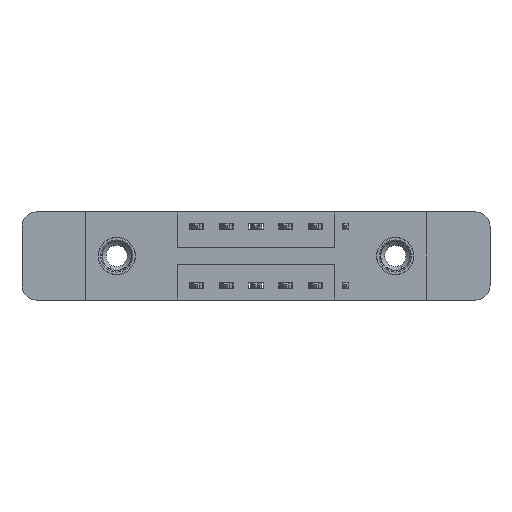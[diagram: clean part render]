
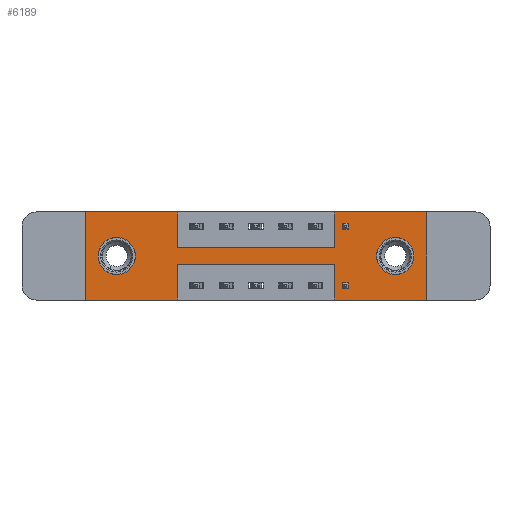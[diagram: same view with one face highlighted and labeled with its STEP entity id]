
A CAD part, front view. The second image highlights one B-rep face of the part: STEP entity #6189.
In plain terms, the highlighted planar face has unit normal (0, -1, 0).
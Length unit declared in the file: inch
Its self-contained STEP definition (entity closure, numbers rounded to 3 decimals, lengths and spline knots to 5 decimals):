
#10 = VERTEX_POINT ( 'NONE', #11869 ) ;
#125 = VECTOR ( 'NONE', #12789, 39.37008 ) ;
#380 = EDGE_CURVE ( 'NONE', #10252, #10491, #4422, .T. ) ;
#447 = EDGE_CURVE ( 'NONE', #5272, #11080, #8510, .T. ) ;
#458 = EDGE_CURVE ( 'NONE', #12099, #11880, #6457, .T. ) ;
#589 = EDGE_CURVE ( 'NONE', #10491, #10252, #1024, .T. ) ;
#596 = ORIENTED_EDGE ( 'NONE', *, *, #3957, .T. ) ;
#652 = CARTESIAN_POINT ( 'NONE',  ( 1.435, 0., -0.37 ) ) ;
#696 = EDGE_LOOP ( 'NONE', ( #4927, #13504, #6667, #5332, #2141, #5871, #3290, #5049, #10887, #3075, #12571, #9923 ) ) ;
#860 = CARTESIAN_POINT ( 'NONE',  ( 1.3025, 0., -0.185 ) ) ;
#926 = CIRCLE ( 'NONE', #1399, 0.078 ) ;
#971 = ORIENTED_EDGE ( 'NONE', *, *, #3456, .T. ) ;
#1024 = CIRCLE ( 'NONE', #1711, 0.078 ) ;
#1135 = CARTESIAN_POINT ( 'NONE',  ( 0.1325, 0., -0.263 ) ) ;
#1215 = VECTOR ( 'NONE', #3801, 39.37008 ) ;
#1244 = CARTESIAN_POINT ( 'NONE',  ( 1.0475, 0., -0.37 ) ) ;
#1246 = AXIS2_PLACEMENT_3D ( 'NONE', #860, #3007, #13574 ) ;
#1248 = CARTESIAN_POINT ( 'NONE',  ( 0., 0., 0. ) ) ;
#1298 = VECTOR ( 'NONE', #4616, 39.37008 ) ;
#1399 = AXIS2_PLACEMENT_3D ( 'NONE', #7793, #7524, #12070 ) ;
#1448 = EDGE_CURVE ( 'NONE', #11471, #2522, #7578, .T. ) ;
#1578 = VERTEX_POINT ( 'NONE', #8200 ) ;
#1674 = CARTESIAN_POINT ( 'NONE',  ( 1.0475, 0., 0. ) ) ;
#1711 = AXIS2_PLACEMENT_3D ( 'NONE', #5689, #4480, #12066 ) ;
#2111 = VECTOR ( 'NONE', #12059, 39.37008 ) ;
#2141 = ORIENTED_EDGE ( 'NONE', *, *, #9659, .F. ) ;
#2290 = DIRECTION ( 'NONE',  ( 0., 0., -1. ) ) ;
#2362 = LINE ( 'NONE', #5828, #8233 ) ;
#2522 = VERTEX_POINT ( 'NONE', #4399 ) ;
#2550 = EDGE_CURVE ( 'NONE', #9935, #12099, #9894, .T. ) ;
#2562 = EDGE_LOOP ( 'NONE', ( #596, #971 ) ) ;
#2643 = VECTOR ( 'NONE', #13912, 39.37008 ) ;
#2678 = VECTOR ( 'NONE', #2910, 39.37008 ) ;
#2857 = VECTOR ( 'NONE', #3156, 39.37008 ) ;
#2876 = EDGE_CURVE ( 'NONE', #11080, #3169, #6768, .T. ) ;
#2910 = DIRECTION ( 'NONE',  ( 0., 0., -1. ) ) ;
#3007 = DIRECTION ( 'NONE',  ( 0., 1., 0. ) ) ;
#3066 = AXIS2_PLACEMENT_3D ( 'NONE', #3286, #5411, #2290 ) ;
#3075 = ORIENTED_EDGE ( 'NONE', *, *, #11669, .F. ) ;
#3156 = DIRECTION ( 'NONE',  ( 0., 0., 1. ) ) ;
#3169 = VERTEX_POINT ( 'NONE', #5979 ) ;
#3219 = DIRECTION ( 'NONE',  ( -1., 0., 0. ) ) ;
#3286 = CARTESIAN_POINT ( 'NONE',  ( 0., 0., -0.37 ) ) ;
#3290 = ORIENTED_EDGE ( 'NONE', *, *, #8631, .F. ) ;
#3338 = VECTOR ( 'NONE', #10888, 39.37008 ) ;
#3456 = EDGE_CURVE ( 'NONE', #3720, #6107, #926, .T. ) ;
#3569 = CARTESIAN_POINT ( 'NONE',  ( 0., 0., -0.37 ) ) ;
#3720 = VERTEX_POINT ( 'NONE', #1135 ) ;
#3801 = DIRECTION ( 'NONE',  ( 1., 0., 0. ) ) ;
#3821 = CARTESIAN_POINT ( 'NONE',  ( 0.1325, 0., -0.185 ) ) ;
#3957 = EDGE_CURVE ( 'NONE', #6107, #3720, #10646, .T. ) ;
#4124 = CARTESIAN_POINT ( 'NONE',  ( 0., 0., -0.37 ) ) ;
#4352 = AXIS2_PLACEMENT_3D ( 'NONE', #3821, #7976, #9968 ) ;
#4399 = CARTESIAN_POINT ( 'NONE',  ( 0.3875, 0., -0.22 ) ) ;
#4422 = CIRCLE ( 'NONE', #1246, 0.078 ) ;
#4480 = DIRECTION ( 'NONE',  ( 0., 1., 0. ) ) ;
#4616 = DIRECTION ( 'NONE',  ( 0., 0., 1. ) ) ;
#4831 = VECTOR ( 'NONE', #10661, 39.37008 ) ;
#4927 = ORIENTED_EDGE ( 'NONE', *, *, #6319, .F. ) ;
#5049 = ORIENTED_EDGE ( 'NONE', *, *, #2876, .F. ) ;
#5078 = DIRECTION ( 'NONE',  ( 0., 0., 1. ) ) ;
#5189 = VECTOR ( 'NONE', #3219, 39.37008 ) ;
#5272 = VERTEX_POINT ( 'NONE', #5586 ) ;
#5332 = ORIENTED_EDGE ( 'NONE', *, *, #10701, .F. ) ;
#5411 = DIRECTION ( 'NONE',  ( 0., -1., 0. ) ) ;
#5586 = CARTESIAN_POINT ( 'NONE',  ( 0.3875, 0., 0. ) ) ;
#5686 = CARTESIAN_POINT ( 'NONE',  ( 1.0475, 0., -0.37 ) ) ;
#5689 = CARTESIAN_POINT ( 'NONE',  ( 1.3025, 0., -0.185 ) ) ;
#5724 = CARTESIAN_POINT ( 'NONE',  ( 0.3875, 0., -0.15 ) ) ;
#5726 = CARTESIAN_POINT ( 'NONE',  ( 1.0475, 0., -0.22 ) ) ;
#5828 = CARTESIAN_POINT ( 'NONE',  ( 0.3875, 0., -0.37 ) ) ;
#5871 = ORIENTED_EDGE ( 'NONE', *, *, #11074, .F. ) ;
#5968 = ORIENTED_EDGE ( 'NONE', *, *, #589, .T. ) ;
#5979 = CARTESIAN_POINT ( 'NONE',  ( 1.0475, 0., -0.15 ) ) ;
#6107 = VERTEX_POINT ( 'NONE', #9718 ) ;
#6189 = ADVANCED_FACE ( 'NONE', ( #12727, #6395, #9641 ), #9776, .T. ) ;
#6319 = EDGE_CURVE ( 'NONE', #2522, #9935, #2362, .T. ) ;
#6395 = FACE_BOUND ( 'NONE', #2562, .T. ) ;
#6409 = CARTESIAN_POINT ( 'NONE',  ( 1.3025, 0., -0.263 ) ) ;
#6457 = LINE ( 'NONE', #10744, #2857 ) ;
#6667 = ORIENTED_EDGE ( 'NONE', *, *, #13720, .F. ) ;
#6722 = LINE ( 'NONE', #5686, #1298 ) ;
#6768 = LINE ( 'NONE', #5724, #1215 ) ;
#7181 = EDGE_LOOP ( 'NONE', ( #5968, #8888 ) ) ;
#7377 = CARTESIAN_POINT ( 'NONE',  ( 0.3875, 0., 0. ) ) ;
#7524 = DIRECTION ( 'NONE',  ( 0., 1., 0. ) ) ;
#7578 = LINE ( 'NONE', #9904, #2111 ) ;
#7610 = LINE ( 'NONE', #1248, #3338 ) ;
#7793 = CARTESIAN_POINT ( 'NONE',  ( 0.1325, 0., -0.185 ) ) ;
#7976 = DIRECTION ( 'NONE',  ( 0., 1., 0. ) ) ;
#8071 = LINE ( 'NONE', #12546, #2678 ) ;
#8200 = CARTESIAN_POINT ( 'NONE',  ( 1.435, 0., 0. ) ) ;
#8233 = VECTOR ( 'NONE', #9991, 39.37008 ) ;
#8510 = LINE ( 'NONE', #7377, #125 ) ;
#8631 = EDGE_CURVE ( 'NONE', #3169, #10, #11256, .T. ) ;
#8888 = ORIENTED_EDGE ( 'NONE', *, *, #380, .T. ) ;
#9162 = VERTEX_POINT ( 'NONE', #652 ) ;
#9641 = FACE_OUTER_BOUND ( 'NONE', #696, .T. ) ;
#9659 = EDGE_CURVE ( 'NONE', #1578, #9162, #8071, .T. ) ;
#9718 = CARTESIAN_POINT ( 'NONE',  ( 0.1325, 0., -0.107 ) ) ;
#9776 = PLANE ( 'NONE',  #3066 ) ;
#9894 = LINE ( 'NONE', #11990, #4831 ) ;
#9904 = CARTESIAN_POINT ( 'NONE',  ( 0.3875, 0., -0.22 ) ) ;
#9923 = ORIENTED_EDGE ( 'NONE', *, *, #2550, .F. ) ;
#9935 = VERTEX_POINT ( 'NONE', #13085 ) ;
#9968 = DIRECTION ( 'NONE',  ( 0., 0., 1. ) ) ;
#9991 = DIRECTION ( 'NONE',  ( 0., 0., -1. ) ) ;
#10252 = VERTEX_POINT ( 'NONE', #6409 ) ;
#10371 = VERTEX_POINT ( 'NONE', #1244 ) ;
#10491 = VERTEX_POINT ( 'NONE', #12153 ) ;
#10551 = LINE ( 'NONE', #4124, #5189 ) ;
#10646 = CIRCLE ( 'NONE', #4352, 0.078 ) ;
#10661 = DIRECTION ( 'NONE',  ( -1., 0., 0. ) ) ;
#10701 = EDGE_CURVE ( 'NONE', #9162, #10371, #10551, .T. ) ;
#10744 = CARTESIAN_POINT ( 'NONE',  ( 0., 0., 0. ) ) ;
#10887 = ORIENTED_EDGE ( 'NONE', *, *, #447, .F. ) ;
#10888 = DIRECTION ( 'NONE',  ( 1., 0., 0. ) ) ;
#11074 = EDGE_CURVE ( 'NONE', #10, #1578, #12629, .T. ) ;
#11080 = VERTEX_POINT ( 'NONE', #11781 ) ;
#11256 = LINE ( 'NONE', #1674, #13363 ) ;
#11471 = VERTEX_POINT ( 'NONE', #5726 ) ;
#11669 = EDGE_CURVE ( 'NONE', #11880, #5272, #7610, .T. ) ;
#11781 = CARTESIAN_POINT ( 'NONE',  ( 0.3875, 0., -0.15 ) ) ;
#11869 = CARTESIAN_POINT ( 'NONE',  ( 1.0475, 0., 0. ) ) ;
#11880 = VERTEX_POINT ( 'NONE', #13798 ) ;
#11990 = CARTESIAN_POINT ( 'NONE',  ( 0., 0., -0.37 ) ) ;
#12059 = DIRECTION ( 'NONE',  ( -1., 0., 0. ) ) ;
#12066 = DIRECTION ( 'NONE',  ( 0., 0., -1. ) ) ;
#12070 = DIRECTION ( 'NONE',  ( 0., 0., 1. ) ) ;
#12099 = VERTEX_POINT ( 'NONE', #3569 ) ;
#12153 = CARTESIAN_POINT ( 'NONE',  ( 1.3025, 0., -0.107 ) ) ;
#12546 = CARTESIAN_POINT ( 'NONE',  ( 1.435, 0., 0. ) ) ;
#12571 = ORIENTED_EDGE ( 'NONE', *, *, #458, .F. ) ;
#12629 = LINE ( 'NONE', #13775, #2643 ) ;
#12727 = FACE_BOUND ( 'NONE', #7181, .T. ) ;
#12789 = DIRECTION ( 'NONE',  ( 0., 0., -1. ) ) ;
#13085 = CARTESIAN_POINT ( 'NONE',  ( 0.3875, 0., -0.37 ) ) ;
#13363 = VECTOR ( 'NONE', #5078, 39.37008 ) ;
#13504 = ORIENTED_EDGE ( 'NONE', *, *, #1448, .F. ) ;
#13574 = DIRECTION ( 'NONE',  ( 0., 0., -1. ) ) ;
#13720 = EDGE_CURVE ( 'NONE', #10371, #11471, #6722, .T. ) ;
#13775 = CARTESIAN_POINT ( 'NONE',  ( 0., 0., 0. ) ) ;
#13798 = CARTESIAN_POINT ( 'NONE',  ( 0., 0., 0. ) ) ;
#13912 = DIRECTION ( 'NONE',  ( 1., 0., 0. ) ) ;
